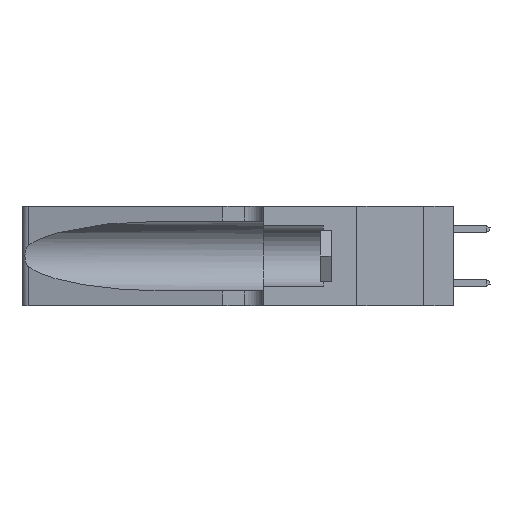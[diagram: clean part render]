
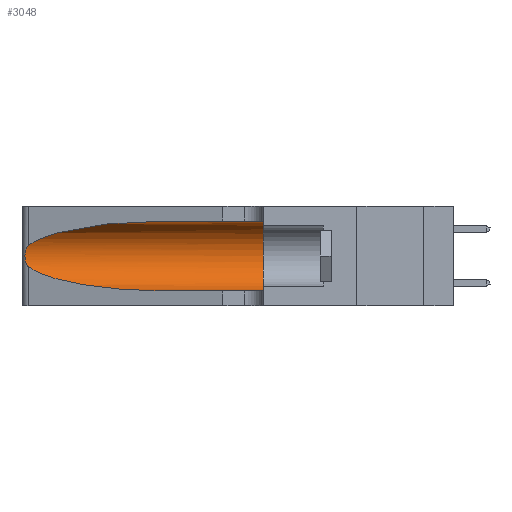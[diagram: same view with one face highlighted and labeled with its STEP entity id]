
A CAD part, left-side view. The second image highlights one B-rep face of the part: STEP entity #3048.
In plain terms, the highlighted cylindrical face has radius 3.308 mm (diameter 6.617 mm), a partial arc.
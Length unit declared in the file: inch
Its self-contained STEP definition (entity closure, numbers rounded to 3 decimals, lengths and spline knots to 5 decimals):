
#370 = ORIENTED_EDGE ( 'NONE', *, *, #1029, .T. ) ;
#838 = CARTESIAN_POINT ( 'NONE',  ( 0.25639, 1.23184, 0.21858 ) ) ;
#1029 = EDGE_CURVE ( 'NONE', #25793, #15003, #25128, .T. ) ;
#1158 = AXIS2_PLACEMENT_3D ( 'NONE', #6622, #10825, #21488 ) ;
#1291 = CARTESIAN_POINT ( 'NONE',  ( 0.1305, 0.72297, 0.31525 ) ) ;
#1390 = DIRECTION ( 'NONE',  ( 0., -1., 0. ) ) ;
#1882 = CARTESIAN_POINT ( 'NONE',  ( 0.1305, 0.72297, 0.05475 ) ) ;
#2919 = VECTOR ( 'NONE', #11539, 39.37008 ) ;
#3048 = ADVANCED_FACE ( 'NONE', ( #4742 ), #15455, .F. ) ;
#3053 = CARTESIAN_POINT ( 'NONE',  ( 0.25854, 1.2359, 0.20912 ) ) ;
#3133 = VERTEX_POINT ( 'NONE', #15420 ) ;
#3248 = ORIENTED_EDGE ( 'NONE', *, *, #8436, .F. ) ;
#3736 = VERTEX_POINT ( 'NONE', #23959 ) ;
#4289 = LINE ( 'NONE', #5762, #15684 ) ;
#4499 = ORIENTED_EDGE ( 'NONE', *, *, #16293, .T. ) ;
#4742 = FACE_OUTER_BOUND ( 'NONE', #20921, .T. ) ;
#4796 = CARTESIAN_POINT ( 'NONE',  ( 0.25487, 1.22718, 0.14631 ) ) ;
#5232 = CARTESIAN_POINT ( 'NONE',  ( 0.26075, 1.23896, 0.19203 ) ) ;
#5544 = DIRECTION ( 'NONE',  ( 0., 1., 0. ) ) ;
#5661 = CARTESIAN_POINT ( 'NONE',  ( 0.25487, 1.22718, 0.22369 ) ) ;
#5762 = CARTESIAN_POINT ( 'NONE',  ( 0.1305, 1.61858, 0.31525 ) ) ;
#5834 = VERTEX_POINT ( 'NONE', #12325 ) ;
#6622 = CARTESIAN_POINT ( 'NONE',  ( 0.1305, 1.61858, 0.185 ) ) ;
#7371 = CARTESIAN_POINT ( 'NONE',  ( 0.26017, 1.23833, 0.17102 ) ) ;
#8436 = EDGE_CURVE ( 'NONE', #3736, #3133, #4289, .T. ) ;
#8714 = CARTESIAN_POINT ( 'NONE',  ( 0.1305, 0.72297, 0.05475 ) ) ;
#8779 = AXIS2_PLACEMENT_3D ( 'NONE', #10336, #5544, #20452 ) ;
#9525 = CARTESIAN_POINT ( 'NONE',  ( 0.25789, 1.23486, 0.15765 ) ) ;
#10336 = CARTESIAN_POINT ( 'NONE',  ( 0.1305, 0.35, 0.185 ) ) ;
#10825 = DIRECTION ( 'NONE',  ( 0., -1., 0. ) ) ;
#11539 = DIRECTION ( 'NONE',  ( 0., -1., 0. ) ) ;
#11672 = CARTESIAN_POINT ( 'NONE',  ( 0.25555, 1.22993, 0.14849 ) ) ;
#12325 = CARTESIAN_POINT ( 'NONE',  ( 0.25487, 1.22718, 0.22369 ) ) ;
#12603 = CARTESIAN_POINT ( 'NONE',  ( 0.18966, 0.96281, 0.05475 ) ) ;
#12703 = EDGE_CURVE ( 'NONE', #3133, #14817, #17444, .T. ) ;
#13609 = ORIENTED_EDGE ( 'NONE', *, *, #23657, .T. ) ;
#13676 = CARTESIAN_POINT ( 'NONE',  ( 0.25555, 1.22994, 0.2215 ) ) ;
#14211 = CARTESIAN_POINT ( 'NONE',  ( 0.18966, 0.96281, 0.31525 ) ) ;
#14356 = LINE ( 'NONE', #24193, #2919 ) ;
#14392 = ORIENTED_EDGE ( 'NONE', *, *, #12703, .F. ) ;
#14546 = EDGE_CURVE ( 'NONE', #15003, #14817, #14356, .T. ) ;
#14817 = VERTEX_POINT ( 'NONE', #27109 ) ;
#15003 = VERTEX_POINT ( 'NONE', #8714 ) ;
#15420 = CARTESIAN_POINT ( 'NONE',  ( 0.1305, 0.35, 0.31525 ) ) ;
#15455 = CYLINDRICAL_SURFACE ( 'NONE', #1158, 0.13025 ) ;
#15684 = VECTOR ( 'NONE', #1390, 39.37008 ) ;
#15915 = CARTESIAN_POINT ( 'NONE',  ( 0.25787, 1.23484, 0.2124 ) ) ;
#16293 = EDGE_CURVE ( 'NONE', #5834, #25793, #27391, .T. ) ;
#16818 = CARTESIAN_POINT ( 'NONE',  ( 0.25487, 1.22718, 0.14631 ) ) ;
#17444 = CIRCLE ( 'NONE', #8779, 0.13025 ) ;
#17615 =( BOUNDED_CURVE ( )  B_SPLINE_CURVE ( 3, ( #1291, #14211, #18480, #5661 ),
 .UNSPECIFIED., .F., .F. ) 
 B_SPLINE_CURVE_WITH_KNOTS ( ( 4, 4 ),
 ( 1.5708, 2.84003 ),
 .UNSPECIFIED. ) 
 CURVE ( )  GEOMETRIC_REPRESENTATION_ITEM ( )  RATIONAL_B_SPLINE_CURVE ( ( 1., 0.87, 0.87, 1. ) ) 
 REPRESENTATION_ITEM ( '' )  );
#18021 = CARTESIAN_POINT ( 'NONE',  ( 0.26018, 1.23835, 0.19895 ) ) ;
#18480 = CARTESIAN_POINT ( 'NONE',  ( 0.2373, 1.15595, 0.28018 ) ) ;
#20043 = CARTESIAN_POINT ( 'NONE',  ( 0.25487, 1.22718, 0.22369 ) ) ;
#20136 = CARTESIAN_POINT ( 'NONE',  ( 0.26075, 1.23896, 0.178 ) ) ;
#20452 = DIRECTION ( 'NONE',  ( 0., 0., 1. ) ) ;
#20921 = EDGE_LOOP ( 'NONE', ( #13609, #4499, #370, #23954, #14392, #3248 ) ) ;
#21488 = DIRECTION ( 'NONE',  ( 0., 0., -1. ) ) ;
#22234 = CARTESIAN_POINT ( 'NONE',  ( 0.25856, 1.23593, 0.16098 ) ) ;
#23657 = EDGE_CURVE ( 'NONE', #3736, #5834, #17615, .T. ) ;
#23954 = ORIENTED_EDGE ( 'NONE', *, *, #14546, .T. ) ;
#23959 = CARTESIAN_POINT ( 'NONE',  ( 0.1305, 0.72297, 0.31525 ) ) ;
#24193 = CARTESIAN_POINT ( 'NONE',  ( 0.1305, 1.61858, 0.05475 ) ) ;
#24319 = CARTESIAN_POINT ( 'NONE',  ( 0.25639, 1.23186, 0.15144 ) ) ;
#25128 =( BOUNDED_CURVE ( )  B_SPLINE_CURVE ( 3, ( #16818, #27234, #12603, #1882 ),
 .UNSPECIFIED., .F., .F. ) 
 B_SPLINE_CURVE_WITH_KNOTS ( ( 4, 4 ),
 ( 3.44316, 4.71239 ),
 .UNSPECIFIED. ) 
 CURVE ( )  GEOMETRIC_REPRESENTATION_ITEM ( )  RATIONAL_B_SPLINE_CURVE ( ( 1., 0.87, 0.87, 1. ) ) 
 REPRESENTATION_ITEM ( '' )  );
#25793 = VERTEX_POINT ( 'NONE', #4796 ) ;
#26363 = CARTESIAN_POINT ( 'NONE',  ( 0.25487, 1.22718, 0.14631 ) ) ;
#27109 = CARTESIAN_POINT ( 'NONE',  ( 0.1305, 0.35, 0.05475 ) ) ;
#27234 = CARTESIAN_POINT ( 'NONE',  ( 0.2373, 1.15595, 0.08982 ) ) ;
#27391 = B_SPLINE_CURVE_WITH_KNOTS ( 'NONE', 3,
 ( #20043, #13676, #838, #15915, #3053, #18021, #5232, #20136, #7371, #22234, #9525, #24319, #11672, #26363 ),
 .UNSPECIFIED., .F., .F.,
 ( 4, 2, 2, 2, 2, 2, 4 ),
 ( 0., 0.00027, 0.00053, 0.00107, 0.0016, 0.00187, 0.00214 ),
 .UNSPECIFIED. ) ;
